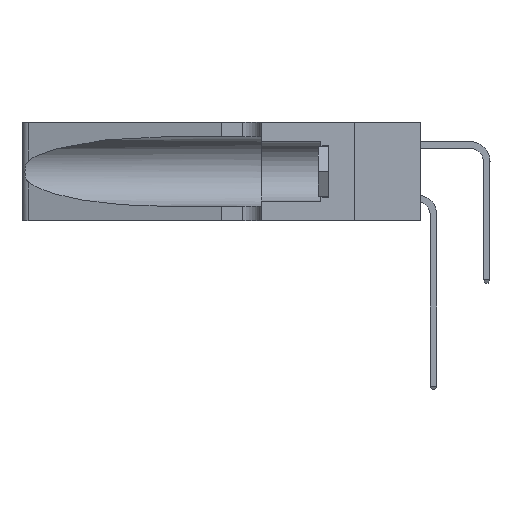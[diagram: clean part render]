
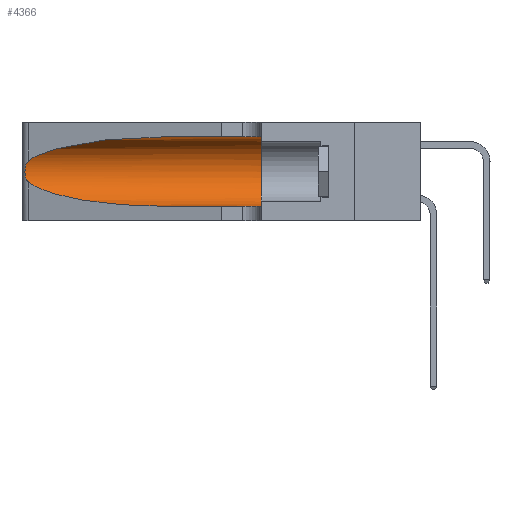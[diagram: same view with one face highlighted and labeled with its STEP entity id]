
A CAD part, left-side view. The second image highlights one B-rep face of the part: STEP entity #4366.
In plain terms, the highlighted cylindrical face has radius 3.308 mm (diameter 6.617 mm), a partial arc.
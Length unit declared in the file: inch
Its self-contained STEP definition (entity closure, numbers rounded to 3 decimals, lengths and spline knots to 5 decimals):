
#662 = VERTEX_POINT ( 'NONE', #10164 ) ;
#700 = CARTESIAN_POINT ( 'NONE',  ( 0.26018, 1.23835, 0.19895 ) ) ;
#1519 = VERTEX_POINT ( 'NONE', #27999 ) ;
#2390 = DIRECTION ( 'NONE',  ( 0., -1., 0. ) ) ;
#3778 = LINE ( 'NONE', #12312, #37728 ) ;
#4076 = CARTESIAN_POINT ( 'NONE',  ( 0.26075, 1.23896, 0.178 ) ) ;
#4107 = ORIENTED_EDGE ( 'NONE', *, *, #12418, .T. ) ;
#4366 = ADVANCED_FACE ( 'NONE', ( #14177 ), #21902, .F. ) ;
#5573 = ORIENTED_EDGE ( 'NONE', *, *, #32443, .F. ) ;
#6019 = CARTESIAN_POINT ( 'NONE',  ( 0.25487, 1.22718, 0.14631 ) ) ;
#6145 = CARTESIAN_POINT ( 'NONE',  ( 0.18966, 0.96281, 0.31525 ) ) ;
#6756 = CARTESIAN_POINT ( 'NONE',  ( 0.25487, 1.22718, 0.22369 ) ) ;
#7446 = CARTESIAN_POINT ( 'NONE',  ( 0.25856, 1.23593, 0.16098 ) ) ;
#7789 = EDGE_CURVE ( 'NONE', #12756, #39110, #37408, .T. ) ;
#7855 = CARTESIAN_POINT ( 'NONE',  ( 0.1305, 0.35, 0.185 ) ) ;
#7924 =( BOUNDED_CURVE ( )  B_SPLINE_CURVE ( 3, ( #23263, #6145, #26495, #6756 ),
 .UNSPECIFIED., .F., .F. ) 
 B_SPLINE_CURVE_WITH_KNOTS ( ( 4, 4 ),
 ( 1.5708, 2.84003 ),
 .UNSPECIFIED. ) 
 CURVE ( )  GEOMETRIC_REPRESENTATION_ITEM ( )  RATIONAL_B_SPLINE_CURVE ( ( 1., 0.87, 0.87, 1. ) ) 
 REPRESENTATION_ITEM ( '' )  );
#9332 = CARTESIAN_POINT ( 'NONE',  ( 0.18966, 0.96281, 0.05475 ) ) ;
#9905 = EDGE_LOOP ( 'NONE', ( #12407, #42481, #4107, #35998, #5573, #15924 ) ) ;
#10164 = CARTESIAN_POINT ( 'NONE',  ( 0.25487, 1.22718, 0.14631 ) ) ;
#10647 = CARTESIAN_POINT ( 'NONE',  ( 0.25487, 1.22718, 0.22369 ) ) ;
#10790 = CARTESIAN_POINT ( 'NONE',  ( 0.25639, 1.23186, 0.15144 ) ) ;
#11203 = DIRECTION ( 'NONE',  ( 0., 0., 1. ) ) ;
#12312 = CARTESIAN_POINT ( 'NONE',  ( 0.1305, 1.61858, 0.31525 ) ) ;
#12407 = ORIENTED_EDGE ( 'NONE', *, *, #14346, .T. ) ;
#12418 = EDGE_CURVE ( 'NONE', #662, #12756, #15668, .T. ) ;
#12756 = VERTEX_POINT ( 'NONE', #24209 ) ;
#14028 = VERTEX_POINT ( 'NONE', #28104 ) ;
#14147 = CARTESIAN_POINT ( 'NONE',  ( 0.25487, 1.22718, 0.14631 ) ) ;
#14177 = FACE_OUTER_BOUND ( 'NONE', #9905, .T. ) ;
#14346 = EDGE_CURVE ( 'NONE', #1519, #14028, #7924, .T. ) ;
#15668 =( BOUNDED_CURVE ( )  B_SPLINE_CURVE ( 3, ( #6019, #29065, #9332, #32339 ),
 .UNSPECIFIED., .F., .F. ) 
 B_SPLINE_CURVE_WITH_KNOTS ( ( 4, 4 ),
 ( 3.44316, 4.71239 ),
 .UNSPECIFIED. ) 
 CURVE ( )  GEOMETRIC_REPRESENTATION_ITEM ( )  RATIONAL_B_SPLINE_CURVE ( ( 1., 0.87, 0.87, 1. ) ) 
 REPRESENTATION_ITEM ( '' )  );
#15924 = ORIENTED_EDGE ( 'NONE', *, *, #17792, .F. ) ;
#16993 = DIRECTION ( 'NONE',  ( 0., -1., 0. ) ) ;
#17300 = CARTESIAN_POINT ( 'NONE',  ( 0.25639, 1.23184, 0.21858 ) ) ;
#17792 = EDGE_CURVE ( 'NONE', #1519, #31530, #3778, .T. ) ;
#20653 = CARTESIAN_POINT ( 'NONE',  ( 0.25854, 1.2359, 0.20912 ) ) ;
#21902 = CYLINDRICAL_SURFACE ( 'NONE', #22628, 0.13025 ) ;
#22628 = AXIS2_PLACEMENT_3D ( 'NONE', #36821, #27138, #40102 ) ;
#23263 = CARTESIAN_POINT ( 'NONE',  ( 0.1305, 0.72297, 0.31525 ) ) ;
#23638 = CARTESIAN_POINT ( 'NONE',  ( 0.1305, 1.61858, 0.05475 ) ) ;
#23937 = CARTESIAN_POINT ( 'NONE',  ( 0.26075, 1.23896, 0.19203 ) ) ;
#24008 = AXIS2_PLACEMENT_3D ( 'NONE', #7855, #30881, #11203 ) ;
#24209 = CARTESIAN_POINT ( 'NONE',  ( 0.1305, 0.72297, 0.05475 ) ) ;
#26495 = CARTESIAN_POINT ( 'NONE',  ( 0.2373, 1.15595, 0.28018 ) ) ;
#27138 = DIRECTION ( 'NONE',  ( 0., -1., 0. ) ) ;
#27185 = CARTESIAN_POINT ( 'NONE',  ( 0.26017, 1.23833, 0.17102 ) ) ;
#27999 = CARTESIAN_POINT ( 'NONE',  ( 0.1305, 0.72297, 0.31525 ) ) ;
#28104 = CARTESIAN_POINT ( 'NONE',  ( 0.25487, 1.22718, 0.22369 ) ) ;
#29065 = CARTESIAN_POINT ( 'NONE',  ( 0.2373, 1.15595, 0.08982 ) ) ;
#30035 = EDGE_CURVE ( 'NONE', #14028, #662, #39733, .T. ) ;
#30336 = CARTESIAN_POINT ( 'NONE',  ( 0.25555, 1.22994, 0.2215 ) ) ;
#30480 = CARTESIAN_POINT ( 'NONE',  ( 0.25789, 1.23486, 0.15765 ) ) ;
#30541 = CARTESIAN_POINT ( 'NONE',  ( 0.1305, 0.35, 0.05475 ) ) ;
#30881 = DIRECTION ( 'NONE',  ( 0., 1., 0. ) ) ;
#31530 = VERTEX_POINT ( 'NONE', #36195 ) ;
#32339 = CARTESIAN_POINT ( 'NONE',  ( 0.1305, 0.72297, 0.05475 ) ) ;
#32443 = EDGE_CURVE ( 'NONE', #31530, #39110, #35113, .T. ) ;
#33742 = CARTESIAN_POINT ( 'NONE',  ( 0.25555, 1.22993, 0.14849 ) ) ;
#35113 = CIRCLE ( 'NONE', #24008, 0.13025 ) ;
#35998 = ORIENTED_EDGE ( 'NONE', *, *, #7789, .T. ) ;
#36195 = CARTESIAN_POINT ( 'NONE',  ( 0.1305, 0.35, 0.31525 ) ) ;
#36410 = VECTOR ( 'NONE', #16993, 39.37008 ) ;
#36821 = CARTESIAN_POINT ( 'NONE',  ( 0.1305, 1.61858, 0.185 ) ) ;
#37408 = LINE ( 'NONE', #23638, #36410 ) ;
#37728 = VECTOR ( 'NONE', #2390, 39.37008 ) ;
#39110 = VERTEX_POINT ( 'NONE', #30541 ) ;
#39733 = B_SPLINE_CURVE_WITH_KNOTS ( 'NONE', 3,
 ( #10647, #30336, #17300, #40150, #20653, #700, #23937, #4076, #27185, #7446, #30480, #10790, #33742, #14147 ),
 .UNSPECIFIED., .F., .F.,
 ( 4, 2, 2, 2, 2, 2, 4 ),
 ( 0., 0.00027, 0.00053, 0.00107, 0.0016, 0.00187, 0.00214 ),
 .UNSPECIFIED. ) ;
#40102 = DIRECTION ( 'NONE',  ( 0., 0., -1. ) ) ;
#40150 = CARTESIAN_POINT ( 'NONE',  ( 0.25787, 1.23484, 0.2124 ) ) ;
#42481 = ORIENTED_EDGE ( 'NONE', *, *, #30035, .T. ) ;
